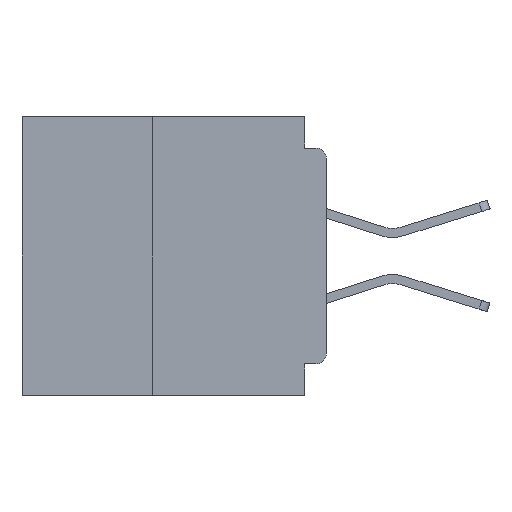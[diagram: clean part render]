
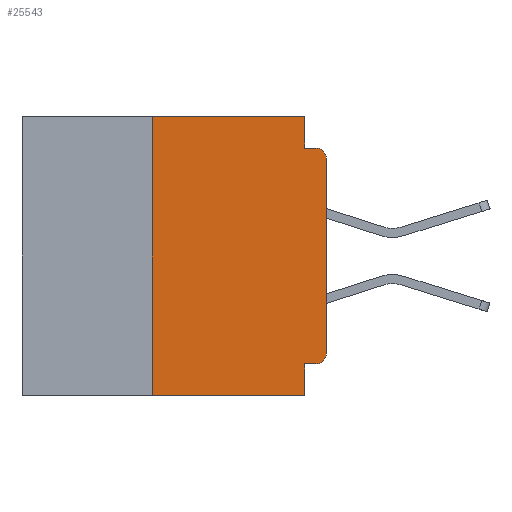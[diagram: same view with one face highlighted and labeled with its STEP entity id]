
A CAD part, left-side view. The second image highlights one B-rep face of the part: STEP entity #25543.
In plain terms, the highlighted planar face has unit normal (-1, 0, 0).
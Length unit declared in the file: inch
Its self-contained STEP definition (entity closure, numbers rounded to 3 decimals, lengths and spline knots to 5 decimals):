
#614 = LINE ( 'NONE', #29397, #8927 ) ;
#1510 = DIRECTION ( 'NONE',  ( 0., 0., -1. ) ) ;
#1540 = VECTOR ( 'NONE', #30373, 39.37008 ) ;
#1605 = LINE ( 'NONE', #45916, #39414 ) ;
#2538 = ORIENTED_EDGE ( 'NONE', *, *, #11095, .F. ) ;
#2645 = LINE ( 'NONE', #30528, #1540 ) ;
#3317 = VERTEX_POINT ( 'NONE', #38174 ) ;
#4129 = AXIS2_PLACEMENT_3D ( 'NONE', #21081, #20973, #20936 ) ;
#4933 = CARTESIAN_POINT ( 'NONE',  ( 0., 0.437, 0. ) ) ;
#4992 = EDGE_CURVE ( 'NONE', #23807, #43176, #9596, .T. ) ;
#5231 = LINE ( 'NONE', #40538, #13571 ) ;
#6063 = EDGE_CURVE ( 'NONE', #3317, #30682, #614, .T. ) ;
#6972 = DIRECTION ( 'NONE',  ( 0., 0., -1. ) ) ;
#6989 = VERTEX_POINT ( 'NONE', #19646 ) ;
#7077 = VECTOR ( 'NONE', #23235, 39.37008 ) ;
#7155 = DIRECTION ( 'NONE',  ( -1., 0., 0. ) ) ;
#8046 = AXIS2_PLACEMENT_3D ( 'NONE', #4933, #22879, #1510 ) ;
#8341 = ORIENTED_EDGE ( 'NONE', *, *, #6063, .F. ) ;
#8927 = VECTOR ( 'NONE', #29693, 39.37008 ) ;
#9596 = CIRCLE ( 'NONE', #4129, 0.015 ) ;
#9924 = VECTOR ( 'NONE', #35403, 39.37008 ) ;
#10114 = ORIENTED_EDGE ( 'NONE', *, *, #32519, .T. ) ;
#10797 = VERTEX_POINT ( 'NONE', #25719 ) ;
#10806 = CARTESIAN_POINT ( 'NONE',  ( 0., 0.015, -0.355 ) ) ;
#10910 = EDGE_CURVE ( 'NONE', #37739, #13855, #5231, .T. ) ;
#11095 = EDGE_CURVE ( 'NONE', #6989, #43176, #41297, .T. ) ;
#12540 = EDGE_CURVE ( 'NONE', #36483, #6989, #1605, .T. ) ;
#12542 = EDGE_CURVE ( 'NONE', #30682, #36483, #38293, .T. ) ;
#12984 = VECTOR ( 'NONE', #41602, 39.37008 ) ;
#13571 = VECTOR ( 'NONE', #44103, 39.37008 ) ;
#13855 = VERTEX_POINT ( 'NONE', #28963 ) ;
#16006 = CARTESIAN_POINT ( 'NONE',  ( 0., 0., -0.06 ) ) ;
#16261 = ORIENTED_EDGE ( 'NONE', *, *, #32556, .T. ) ;
#16802 = CARTESIAN_POINT ( 'NONE',  ( 0., 0., -0.045 ) ) ;
#17365 = CARTESIAN_POINT ( 'NONE',  ( 0., 0., -0.34 ) ) ;
#19288 = PLANE ( 'NONE',  #8046 ) ;
#19646 = CARTESIAN_POINT ( 'NONE',  ( 0., 0.031, -0.045 ) ) ;
#19660 = CARTESIAN_POINT ( 'NONE',  ( 0., 0.031, -0.4 ) ) ;
#19680 = CIRCLE ( 'NONE', #43119, 0.015 ) ;
#20152 = ORIENTED_EDGE ( 'NONE', *, *, #12540, .F. ) ;
#20789 = VECTOR ( 'NONE', #21212, 39.37008 ) ;
#20936 = DIRECTION ( 'NONE',  ( 0., 0., -1. ) ) ;
#20973 = DIRECTION ( 'NONE',  ( -1., 0., 0. ) ) ;
#21081 = CARTESIAN_POINT ( 'NONE',  ( 0., 0.015, -0.06 ) ) ;
#21212 = DIRECTION ( 'NONE',  ( 0., 0., 1. ) ) ;
#21395 = FACE_OUTER_BOUND ( 'NONE', #45135, .T. ) ;
#22879 = DIRECTION ( 'NONE',  ( 1., 0., 0. ) ) ;
#23235 = DIRECTION ( 'NONE',  ( 0., 0., -1. ) ) ;
#23807 = VERTEX_POINT ( 'NONE', #16006 ) ;
#25543 = ADVANCED_FACE ( 'NONE', ( #21395 ), #19288, .F. ) ;
#25719 = CARTESIAN_POINT ( 'NONE',  ( 0., 0.031, -0.4 ) ) ;
#27144 = ORIENTED_EDGE ( 'NONE', *, *, #12542, .F. ) ;
#28481 = CARTESIAN_POINT ( 'NONE',  ( 0., 0.015, -0.34 ) ) ;
#28848 = EDGE_CURVE ( 'NONE', #3317, #10797, #2645, .T. ) ;
#28963 = CARTESIAN_POINT ( 'NONE',  ( 0., 0.031, -0.355 ) ) ;
#29397 = CARTESIAN_POINT ( 'NONE',  ( 0., 0.25, -0.4 ) ) ;
#29693 = DIRECTION ( 'NONE',  ( 0., 0., 1. ) ) ;
#30003 = VERTEX_POINT ( 'NONE', #17365 ) ;
#30187 = LINE ( 'NONE', #42400, #20789 ) ;
#30373 = DIRECTION ( 'NONE',  ( 0., -1., 0. ) ) ;
#30528 = CARTESIAN_POINT ( 'NONE',  ( 0., 0.437, -0.4 ) ) ;
#30682 = VERTEX_POINT ( 'NONE', #31695 ) ;
#31118 = ORIENTED_EDGE ( 'NONE', *, *, #4992, .T. ) ;
#31695 = CARTESIAN_POINT ( 'NONE',  ( 0., 0.25, 0. ) ) ;
#31823 = CARTESIAN_POINT ( 'NONE',  ( 0., 0.437, 0. ) ) ;
#32008 = DIRECTION ( 'NONE',  ( 0., 0., -1. ) ) ;
#32361 = ORIENTED_EDGE ( 'NONE', *, *, #10910, .F. ) ;
#32519 = EDGE_CURVE ( 'NONE', #30003, #23807, #30187, .T. ) ;
#32556 = EDGE_CURVE ( 'NONE', #37739, #30003, #19680, .T. ) ;
#34795 = CARTESIAN_POINT ( 'NONE',  ( 0., 0.015, -0.045 ) ) ;
#35403 = DIRECTION ( 'NONE',  ( 0., -1., 0. ) ) ;
#35436 = LINE ( 'NONE', #19660, #7077 ) ;
#36483 = VERTEX_POINT ( 'NONE', #42421 ) ;
#37739 = VERTEX_POINT ( 'NONE', #10806 ) ;
#38174 = CARTESIAN_POINT ( 'NONE',  ( 0., 0.25, -0.4 ) ) ;
#38293 = LINE ( 'NONE', #31823, #9924 ) ;
#38322 = ORIENTED_EDGE ( 'NONE', *, *, #28848, .T. ) ;
#39414 = VECTOR ( 'NONE', #6972, 39.37008 ) ;
#40511 = EDGE_CURVE ( 'NONE', #13855, #10797, #35436, .T. ) ;
#40538 = CARTESIAN_POINT ( 'NONE',  ( 0., 0., -0.355 ) ) ;
#41297 = LINE ( 'NONE', #16802, #12984 ) ;
#41602 = DIRECTION ( 'NONE',  ( 0., -1., 0. ) ) ;
#42273 = ORIENTED_EDGE ( 'NONE', *, *, #40511, .F. ) ;
#42400 = CARTESIAN_POINT ( 'NONE',  ( 0., 0., 0. ) ) ;
#42421 = CARTESIAN_POINT ( 'NONE',  ( 0., 0.031, 0. ) ) ;
#43119 = AXIS2_PLACEMENT_3D ( 'NONE', #28481, #7155, #32008 ) ;
#43176 = VERTEX_POINT ( 'NONE', #34795 ) ;
#44103 = DIRECTION ( 'NONE',  ( 0., 1., 0. ) ) ;
#45135 = EDGE_LOOP ( 'NONE', ( #10114, #31118, #2538, #20152, #27144, #8341, #38322, #42273, #32361, #16261 ) ) ;
#45916 = CARTESIAN_POINT ( 'NONE',  ( 0., 0.031, 0. ) ) ;
